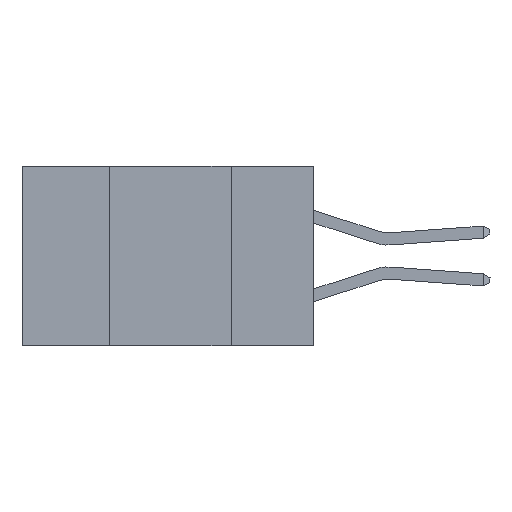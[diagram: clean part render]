
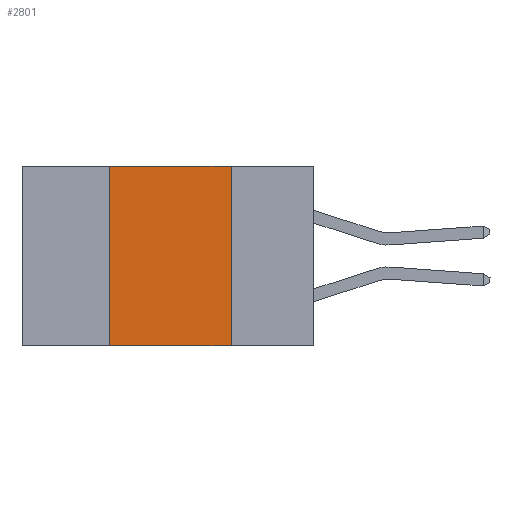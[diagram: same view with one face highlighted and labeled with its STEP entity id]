
A CAD part, left-side view. The second image highlights one B-rep face of the part: STEP entity #2801.
In plain terms, the highlighted planar face has unit normal (-1, 0, 0).
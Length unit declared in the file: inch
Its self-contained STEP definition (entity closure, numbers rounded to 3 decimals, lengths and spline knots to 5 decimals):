
#950 = VECTOR ( 'NONE', #3809, 39.37008 ) ;
#1315 = LINE ( 'NONE', #11392, #950 ) ;
#1694 = ORIENTED_EDGE ( 'NONE', *, *, #12483, .F. ) ;
#1809 = CARTESIAN_POINT ( 'NONE',  ( 0., 0.6, -0.37 ) ) ;
#2180 = CARTESIAN_POINT ( 'NONE',  ( 0., 0.42, 0. ) ) ;
#2801 = ADVANCED_FACE ( 'NONE', ( #11567 ), #7198, .F. ) ;
#3126 = LINE ( 'NONE', #4419, #11774 ) ;
#3809 = DIRECTION ( 'NONE',  ( 0., -1., 0. ) ) ;
#4419 = CARTESIAN_POINT ( 'NONE',  ( 0., 0.17, 0. ) ) ;
#4426 = VERTEX_POINT ( 'NONE', #10743 ) ;
#5393 = ORIENTED_EDGE ( 'NONE', *, *, #13464, .T. ) ;
#5867 = CARTESIAN_POINT ( 'NONE',  ( 0., 0.42, -0.37 ) ) ;
#7119 = DIRECTION ( 'NONE',  ( 0., 0., -1. ) ) ;
#7147 = DIRECTION ( 'NONE',  ( 1., 0., 0. ) ) ;
#7193 = CARTESIAN_POINT ( 'NONE',  ( 0., 0.6, 0. ) ) ;
#7198 = PLANE ( 'NONE',  #12992 ) ;
#8134 = CARTESIAN_POINT ( 'NONE',  ( 0., 0.42, 0. ) ) ;
#8868 = DIRECTION ( 'NONE',  ( 0., 0., 1. ) ) ;
#8958 = VERTEX_POINT ( 'NONE', #8134 ) ;
#9433 = EDGE_LOOP ( 'NONE', ( #10032, #13040, #1694, #5393 ) ) ;
#9526 = VERTEX_POINT ( 'NONE', #5867 ) ;
#9530 = LINE ( 'NONE', #2180, #13493 ) ;
#10032 = ORIENTED_EDGE ( 'NONE', *, *, #11775, .F. ) ;
#10743 = CARTESIAN_POINT ( 'NONE',  ( 0., 0.17, -0.37 ) ) ;
#10994 = VECTOR ( 'NONE', #11701, 39.37008 ) ;
#11392 = CARTESIAN_POINT ( 'NONE',  ( 0., 0.6, 0. ) ) ;
#11567 = FACE_OUTER_BOUND ( 'NONE', #9433, .T. ) ;
#11701 = DIRECTION ( 'NONE',  ( 0., -1., 0. ) ) ;
#11774 = VECTOR ( 'NONE', #11953, 39.37008 ) ;
#11775 = EDGE_CURVE ( 'NONE', #11996, #4426, #3126, .T. ) ;
#11953 = DIRECTION ( 'NONE',  ( 0., 0., -1. ) ) ;
#11996 = VERTEX_POINT ( 'NONE', #12271 ) ;
#12096 = EDGE_CURVE ( 'NONE', #8958, #11996, #1315, .T. ) ;
#12271 = CARTESIAN_POINT ( 'NONE',  ( 0., 0.17, 0. ) ) ;
#12483 = EDGE_CURVE ( 'NONE', #9526, #8958, #9530, .T. ) ;
#12992 = AXIS2_PLACEMENT_3D ( 'NONE', #7193, #7147, #7119 ) ;
#13040 = ORIENTED_EDGE ( 'NONE', *, *, #12096, .F. ) ;
#13464 = EDGE_CURVE ( 'NONE', #9526, #4426, #13471, .T. ) ;
#13471 = LINE ( 'NONE', #1809, #10994 ) ;
#13493 = VECTOR ( 'NONE', #8868, 39.37008 ) ;
